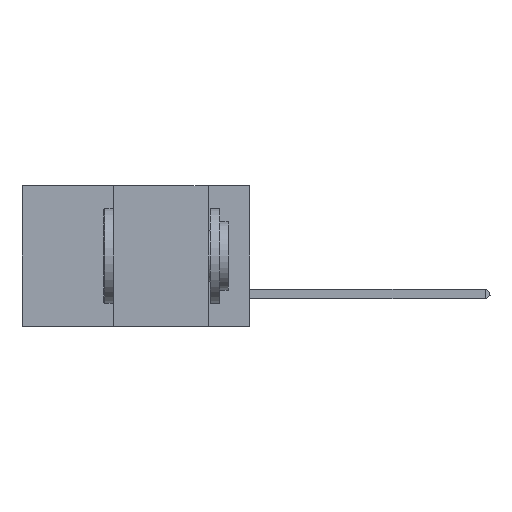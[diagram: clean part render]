
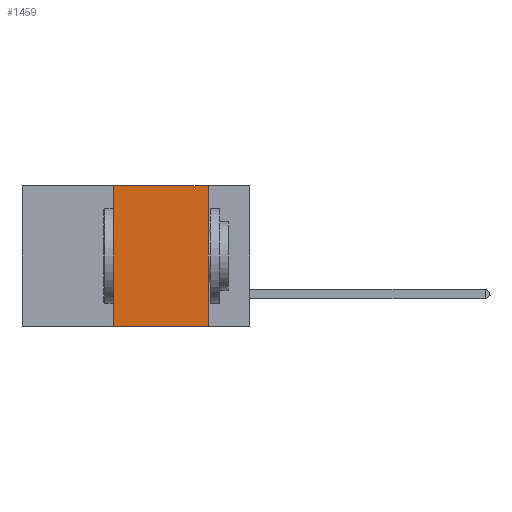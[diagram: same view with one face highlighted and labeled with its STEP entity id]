
A CAD part, left-side view. The second image highlights one B-rep face of the part: STEP entity #1459.
In plain terms, the highlighted planar face has unit normal (-1, 0, 0).
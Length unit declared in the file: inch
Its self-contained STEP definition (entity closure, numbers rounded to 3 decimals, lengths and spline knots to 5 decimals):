
#607 = CARTESIAN_POINT ( 'NONE',  ( 0., 0.36, -0.37 ) ) ;
#1331 = CARTESIAN_POINT ( 'NONE',  ( 0., 0.11, 0. ) ) ;
#1459 = ADVANCED_FACE ( 'NONE', ( #1778 ), #10458, .F. ) ;
#1778 = FACE_OUTER_BOUND ( 'NONE', #2200, .T. ) ;
#2200 = EDGE_LOOP ( 'NONE', ( #7813, #6225, #14258, #20111 ) ) ;
#2257 = CARTESIAN_POINT ( 'NONE',  ( 0., 0.6, 0. ) ) ;
#2647 = VECTOR ( 'NONE', #4442, 39.37008 ) ;
#3349 = CARTESIAN_POINT ( 'NONE',  ( 0., 0.36, 0. ) ) ;
#4442 = DIRECTION ( 'NONE',  ( 0., 0., -1. ) ) ;
#4813 = CARTESIAN_POINT ( 'NONE',  ( 0., 0.36, 0. ) ) ;
#4994 = DIRECTION ( 'NONE',  ( 0., 0., 1. ) ) ;
#6225 = ORIENTED_EDGE ( 'NONE', *, *, #22824, .F. ) ;
#6598 = EDGE_CURVE ( 'NONE', #9628, #11186, #14612, .T. ) ;
#6692 = LINE ( 'NONE', #21037, #10055 ) ;
#7732 = CARTESIAN_POINT ( 'NONE',  ( 0., 0.11, -0.37 ) ) ;
#7813 = ORIENTED_EDGE ( 'NONE', *, *, #6598, .F. ) ;
#8845 = VERTEX_POINT ( 'NONE', #4813 ) ;
#9628 = VERTEX_POINT ( 'NONE', #1331 ) ;
#10055 = VECTOR ( 'NONE', #22955, 39.37008 ) ;
#10211 = EDGE_CURVE ( 'NONE', #13244, #8845, #17249, .T. ) ;
#10458 = PLANE ( 'NONE',  #19587 ) ;
#11186 = VERTEX_POINT ( 'NONE', #7732 ) ;
#12054 = DIRECTION ( 'NONE',  ( 0., 0., -1. ) ) ;
#13244 = VERTEX_POINT ( 'NONE', #607 ) ;
#13281 = LINE ( 'NONE', #2257, #16599 ) ;
#13733 = CARTESIAN_POINT ( 'NONE',  ( 0., 0.11, 0. ) ) ;
#14258 = ORIENTED_EDGE ( 'NONE', *, *, #10211, .F. ) ;
#14612 = LINE ( 'NONE', #13733, #2647 ) ;
#16599 = VECTOR ( 'NONE', #18227, 39.37008 ) ;
#17249 = LINE ( 'NONE', #3349, #17517 ) ;
#17517 = VECTOR ( 'NONE', #4994, 39.37008 ) ;
#17861 = EDGE_CURVE ( 'NONE', #13244, #11186, #6692, .T. ) ;
#18227 = DIRECTION ( 'NONE',  ( 0., -1., 0. ) ) ;
#19587 = AXIS2_PLACEMENT_3D ( 'NONE', #22939, #23019, #12054 ) ;
#20111 = ORIENTED_EDGE ( 'NONE', *, *, #17861, .T. ) ;
#21037 = CARTESIAN_POINT ( 'NONE',  ( 0., 0.6, -0.37 ) ) ;
#22824 = EDGE_CURVE ( 'NONE', #8845, #9628, #13281, .T. ) ;
#22939 = CARTESIAN_POINT ( 'NONE',  ( 0., 0.6, 0. ) ) ;
#22955 = DIRECTION ( 'NONE',  ( 0., -1., 0. ) ) ;
#23019 = DIRECTION ( 'NONE',  ( 1., 0., 0. ) ) ;
